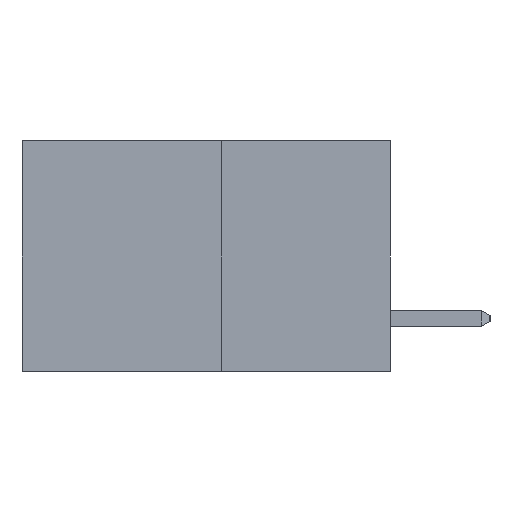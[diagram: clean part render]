
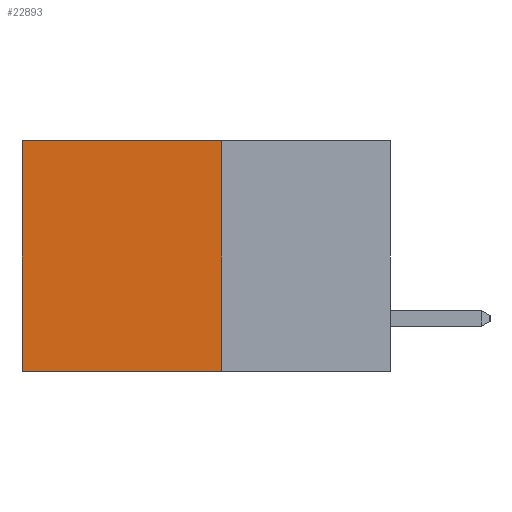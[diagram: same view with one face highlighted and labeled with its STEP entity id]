
A CAD part, left-side view. The second image highlights one B-rep face of the part: STEP entity #22893.
In plain terms, the highlighted planar face has unit normal (-1, 0, 0).
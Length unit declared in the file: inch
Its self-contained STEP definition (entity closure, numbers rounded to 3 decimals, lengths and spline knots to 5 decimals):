
#977 = VERTEX_POINT ( 'NONE', #19850 ) ;
#1286 = DIRECTION ( 'NONE',  ( 1., 0., 0. ) ) ;
#1741 = FACE_OUTER_BOUND ( 'NONE', #16995, .T. ) ;
#3077 = VECTOR ( 'NONE', #20917, 39.37008 ) ;
#3572 = VECTOR ( 'NONE', #20459, 39.37008 ) ;
#5216 = ORIENTED_EDGE ( 'NONE', *, *, #13721, .F. ) ;
#5973 = CARTESIAN_POINT ( 'NONE',  ( 0.277, 0.27, -0.37 ) ) ;
#6644 = VECTOR ( 'NONE', #11423, 39.37008 ) ;
#8213 = ORIENTED_EDGE ( 'NONE', *, *, #22443, .F. ) ;
#8914 = CARTESIAN_POINT ( 'NONE',  ( 0.277, 0.27, 0. ) ) ;
#9261 = CARTESIAN_POINT ( 'NONE',  ( 0.277, 0.27, 0. ) ) ;
#9792 = CARTESIAN_POINT ( 'NONE',  ( 0.277, 0.59, -0.37 ) ) ;
#11423 = DIRECTION ( 'NONE',  ( 0., 1., 0. ) ) ;
#12849 = ORIENTED_EDGE ( 'NONE', *, *, #26377, .T. ) ;
#13119 = EDGE_CURVE ( 'NONE', #21326, #16587, #18672, .T. ) ;
#13608 = DIRECTION ( 'NONE',  ( 0., 0., -1. ) ) ;
#13721 = EDGE_CURVE ( 'NONE', #21326, #26350, #20296, .T. ) ;
#13768 = LINE ( 'NONE', #5973, #3077 ) ;
#13822 = AXIS2_PLACEMENT_3D ( 'NONE', #14068, #1286, #16217 ) ;
#13927 = VECTOR ( 'NONE', #13608, 39.37008 ) ;
#14003 = CARTESIAN_POINT ( 'NONE',  ( 0.277, 0.27, -0.37 ) ) ;
#14068 = CARTESIAN_POINT ( 'NONE',  ( 0.277, 0.27, -0.37 ) ) ;
#16217 = DIRECTION ( 'NONE',  ( 0., 0., -1. ) ) ;
#16587 = VERTEX_POINT ( 'NONE', #23956 ) ;
#16995 = EDGE_LOOP ( 'NONE', ( #12849, #8213, #5216, #22227 ) ) ;
#17946 = CARTESIAN_POINT ( 'NONE',  ( 0.277, 0.27, -0.37 ) ) ;
#18672 = LINE ( 'NONE', #9261, #6644 ) ;
#19850 = CARTESIAN_POINT ( 'NONE',  ( 0.277, 0.59, -0.37 ) ) ;
#20296 = LINE ( 'NONE', #17946, #13927 ) ;
#20459 = DIRECTION ( 'NONE',  ( 0., 0., -1. ) ) ;
#20598 = LINE ( 'NONE', #9792, #3572 ) ;
#20917 = DIRECTION ( 'NONE',  ( 0., 1., 0. ) ) ;
#21326 = VERTEX_POINT ( 'NONE', #8914 ) ;
#22227 = ORIENTED_EDGE ( 'NONE', *, *, #13119, .T. ) ;
#22443 = EDGE_CURVE ( 'NONE', #26350, #977, #13768, .T. ) ;
#22581 = PLANE ( 'NONE',  #13822 ) ;
#22893 = ADVANCED_FACE ( 'NONE', ( #1741 ), #22581, .F. ) ;
#23956 = CARTESIAN_POINT ( 'NONE',  ( 0.277, 0.59, 0. ) ) ;
#26350 = VERTEX_POINT ( 'NONE', #14003 ) ;
#26377 = EDGE_CURVE ( 'NONE', #16587, #977, #20598, .T. ) ;
